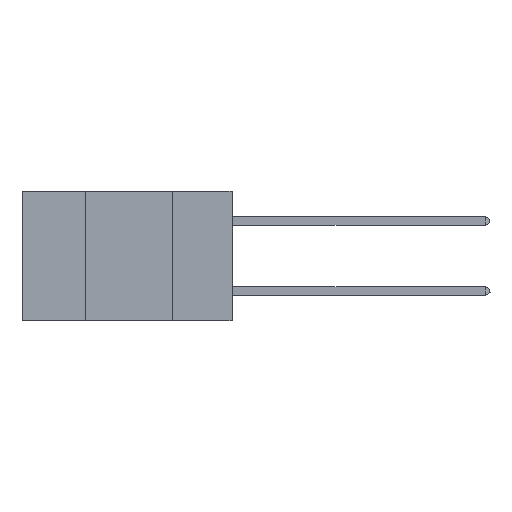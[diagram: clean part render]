
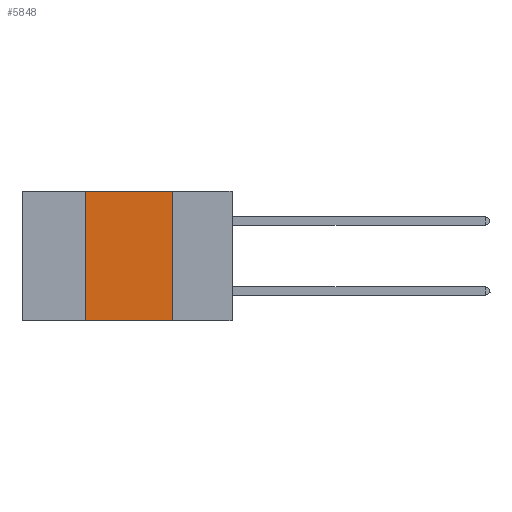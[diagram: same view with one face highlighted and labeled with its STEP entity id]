
A CAD part, left-side view. The second image highlights one B-rep face of the part: STEP entity #5848.
In plain terms, the highlighted planar face has unit normal (-1, 0, 0).
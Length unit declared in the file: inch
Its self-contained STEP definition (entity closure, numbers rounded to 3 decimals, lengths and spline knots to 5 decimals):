
#302 = EDGE_LOOP ( 'NONE', ( #12743, #8697, #10468, #8544 ) ) ;
#351 = VERTEX_POINT ( 'NONE', #1346 ) ;
#678 = DIRECTION ( 'NONE',  ( 0., 0., -1. ) ) ;
#1346 = CARTESIAN_POINT ( 'NONE',  ( 0., 0.42, -0.37 ) ) ;
#1814 = CARTESIAN_POINT ( 'NONE',  ( 0., 0.6, 0. ) ) ;
#2273 = DIRECTION ( 'NONE',  ( 0., 0., 1. ) ) ;
#2384 = VERTEX_POINT ( 'NONE', #7934 ) ;
#2960 = AXIS2_PLACEMENT_3D ( 'NONE', #1814, #6482, #678 ) ;
#2998 = EDGE_CURVE ( 'NONE', #351, #5526, #10296, .T. ) ;
#3020 = CARTESIAN_POINT ( 'NONE',  ( 0., 0.6, 0. ) ) ;
#4421 = LINE ( 'NONE', #3020, #14675 ) ;
#4643 = EDGE_CURVE ( 'NONE', #351, #2384, #13836, .T. ) ;
#4861 = LINE ( 'NONE', #15327, #9310 ) ;
#5526 = VERTEX_POINT ( 'NONE', #10600 ) ;
#5848 = ADVANCED_FACE ( 'NONE', ( #7735 ), #12643, .F. ) ;
#6482 = DIRECTION ( 'NONE',  ( 1., 0., 0. ) ) ;
#6882 = CARTESIAN_POINT ( 'NONE',  ( 0., 0.42, 0. ) ) ;
#7133 = VECTOR ( 'NONE', #14131, 39.37008 ) ;
#7289 = CARTESIAN_POINT ( 'NONE',  ( 0., 0.17, 0. ) ) ;
#7620 = VERTEX_POINT ( 'NONE', #7289 ) ;
#7735 = FACE_OUTER_BOUND ( 'NONE', #302, .T. ) ;
#7934 = CARTESIAN_POINT ( 'NONE',  ( 0., 0.42, 0. ) ) ;
#8021 = EDGE_CURVE ( 'NONE', #7620, #5526, #4861, .T. ) ;
#8407 = VECTOR ( 'NONE', #2273, 39.37008 ) ;
#8544 = ORIENTED_EDGE ( 'NONE', *, *, #2998, .T. ) ;
#8697 = ORIENTED_EDGE ( 'NONE', *, *, #9583, .F. ) ;
#9310 = VECTOR ( 'NONE', #11896, 39.37008 ) ;
#9583 = EDGE_CURVE ( 'NONE', #2384, #7620, #4421, .T. ) ;
#10296 = LINE ( 'NONE', #11723, #7133 ) ;
#10468 = ORIENTED_EDGE ( 'NONE', *, *, #4643, .F. ) ;
#10600 = CARTESIAN_POINT ( 'NONE',  ( 0., 0.17, -0.37 ) ) ;
#11153 = DIRECTION ( 'NONE',  ( 0., -1., 0. ) ) ;
#11723 = CARTESIAN_POINT ( 'NONE',  ( 0., 0.6, -0.37 ) ) ;
#11896 = DIRECTION ( 'NONE',  ( 0., 0., -1. ) ) ;
#12643 = PLANE ( 'NONE',  #2960 ) ;
#12743 = ORIENTED_EDGE ( 'NONE', *, *, #8021, .F. ) ;
#13836 = LINE ( 'NONE', #6882, #8407 ) ;
#14131 = DIRECTION ( 'NONE',  ( 0., -1., 0. ) ) ;
#14675 = VECTOR ( 'NONE', #11153, 39.37008 ) ;
#15327 = CARTESIAN_POINT ( 'NONE',  ( 0., 0.17, 0. ) ) ;
